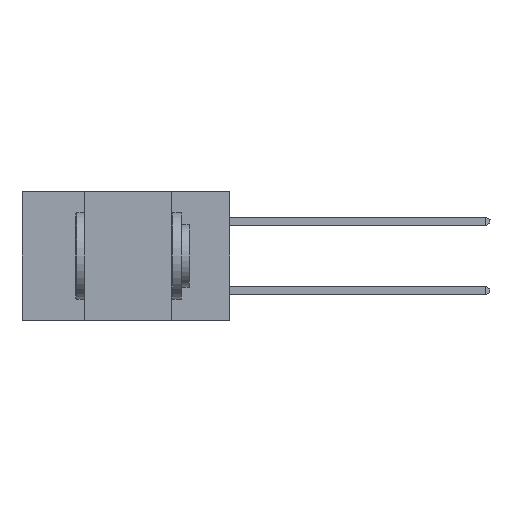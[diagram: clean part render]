
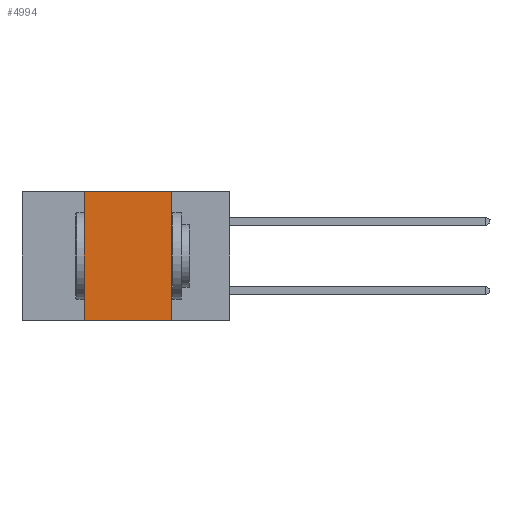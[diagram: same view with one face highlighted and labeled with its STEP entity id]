
A CAD part, left-side view. The second image highlights one B-rep face of the part: STEP entity #4994.
In plain terms, the highlighted planar face has unit normal (-1, 0, 0).
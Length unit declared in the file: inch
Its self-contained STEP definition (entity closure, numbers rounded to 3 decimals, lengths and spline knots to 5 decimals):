
#542 = DIRECTION ( 'NONE',  ( 0., -1., 0. ) ) ;
#604 = CARTESIAN_POINT ( 'NONE',  ( 0., 0.6, -0.37 ) ) ;
#1317 = VECTOR ( 'NONE', #6937, 39.37008 ) ;
#1318 = EDGE_CURVE ( 'NONE', #18838, #23433, #2565, .T. ) ;
#1385 = ORIENTED_EDGE ( 'NONE', *, *, #18821, .F. ) ;
#2565 = LINE ( 'NONE', #22630, #21137 ) ;
#2703 = VECTOR ( 'NONE', #20011, 39.37008 ) ;
#2775 = CARTESIAN_POINT ( 'NONE',  ( 0., 0.17, -0.37 ) ) ;
#3399 = DIRECTION ( 'NONE',  ( 0., 0., -1. ) ) ;
#3497 = CARTESIAN_POINT ( 'NONE',  ( 0., 0.42, -0.37 ) ) ;
#4994 = ADVANCED_FACE ( 'NONE', ( #5424 ), #7719, .F. ) ;
#5233 = CARTESIAN_POINT ( 'NONE',  ( 0., 0.42, 0. ) ) ;
#5424 = FACE_OUTER_BOUND ( 'NONE', #19369, .T. ) ;
#6715 = VECTOR ( 'NONE', #26905, 39.37008 ) ;
#6937 = DIRECTION ( 'NONE',  ( 0., 0., -1. ) ) ;
#7719 = PLANE ( 'NONE',  #20827 ) ;
#10291 = CARTESIAN_POINT ( 'NONE',  ( 0., 0.6, 0. ) ) ;
#10783 = VERTEX_POINT ( 'NONE', #3497 ) ;
#12409 = EDGE_CURVE ( 'NONE', #10783, #21356, #21321, .T. ) ;
#12438 = EDGE_CURVE ( 'NONE', #23433, #21356, #15552, .T. ) ;
#13274 = CARTESIAN_POINT ( 'NONE',  ( 0., 0.17, -0.37 ) ) ;
#14803 = LINE ( 'NONE', #18169, #6715 ) ;
#15552 = LINE ( 'NONE', #2775, #1317 ) ;
#16205 = ORIENTED_EDGE ( 'NONE', *, *, #1318, .F. ) ;
#16820 = ORIENTED_EDGE ( 'NONE', *, *, #12438, .F. ) ;
#17366 = CARTESIAN_POINT ( 'NONE',  ( 0., 0.17, 0. ) ) ;
#18169 = CARTESIAN_POINT ( 'NONE',  ( 0., 0.42, -0.37 ) ) ;
#18821 = EDGE_CURVE ( 'NONE', #10783, #18838, #14803, .T. ) ;
#18838 = VERTEX_POINT ( 'NONE', #5233 ) ;
#19042 = DIRECTION ( 'NONE',  ( 1., 0., 0. ) ) ;
#19369 = EDGE_LOOP ( 'NONE', ( #16820, #16205, #1385, #26773 ) ) ;
#20011 = DIRECTION ( 'NONE',  ( 0., -1., 0. ) ) ;
#20827 = AXIS2_PLACEMENT_3D ( 'NONE', #10291, #19042, #3399 ) ;
#21137 = VECTOR ( 'NONE', #542, 39.37008 ) ;
#21321 = LINE ( 'NONE', #604, #2703 ) ;
#21356 = VERTEX_POINT ( 'NONE', #13274 ) ;
#22630 = CARTESIAN_POINT ( 'NONE',  ( 0., 0.6, 0. ) ) ;
#23433 = VERTEX_POINT ( 'NONE', #17366 ) ;
#26773 = ORIENTED_EDGE ( 'NONE', *, *, #12409, .T. ) ;
#26905 = DIRECTION ( 'NONE',  ( 0., 0., 1. ) ) ;
